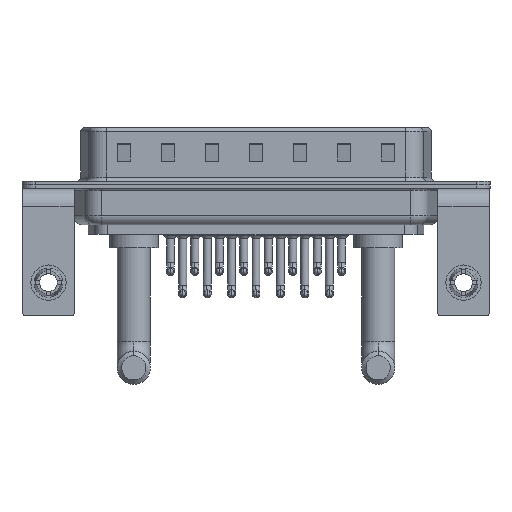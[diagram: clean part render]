
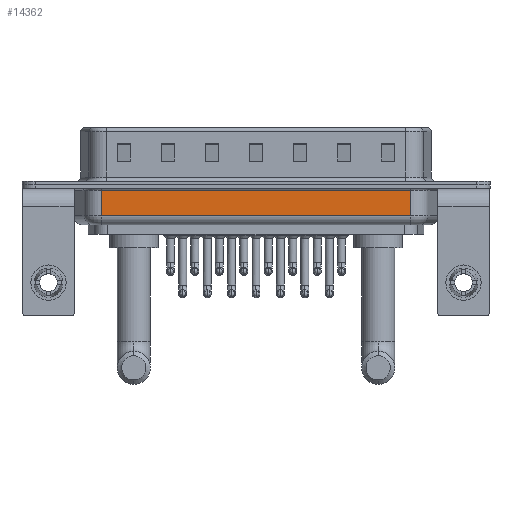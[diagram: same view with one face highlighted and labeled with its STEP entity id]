
A CAD part, front view. The second image highlights one B-rep face of the part: STEP entity #14362.
In plain terms, the highlighted planar face has unit normal (0, -1, 0).
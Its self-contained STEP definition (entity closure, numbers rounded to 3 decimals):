
#244 = CARTESIAN_POINT ( 'NONE',  ( 41.044, -5.35, -4.5 ) ) ;
#3924 = DIRECTION ( 'NONE',  ( 1., 0., 0. ) ) ;
#5867 = EDGE_CURVE ( 'NONE', #6937, #7468, #16823, .T. ) ;
#6099 = CARTESIAN_POINT ( 'NONE',  ( 6.006, -5.35, -3.5 ) ) ;
#6937 = VERTEX_POINT ( 'NONE', #19471 ) ;
#7468 = VERTEX_POINT ( 'NONE', #15445 ) ;
#7800 = LINE ( 'NONE', #26986, #19306 ) ;
#8134 = DIRECTION ( 'NONE',  ( -1., 0., 0. ) ) ;
#8943 = VECTOR ( 'NONE', #19300, 1000. ) ;
#9081 = EDGE_CURVE ( 'NONE', #18091, #7468, #10720, .T. ) ;
#10141 = AXIS2_PLACEMENT_3D ( 'NONE', #13619, #23970, #24506 ) ;
#10152 = CARTESIAN_POINT ( 'NONE',  ( 41.044, -5.35, -3.5 ) ) ;
#10720 = LINE ( 'NONE', #19139, #20099 ) ;
#12182 = ORIENTED_EDGE ( 'NONE', *, *, #18726, .T. ) ;
#13619 = CARTESIAN_POINT ( 'NONE',  ( 6.006, -5.35, -4.5 ) ) ;
#14362 = ADVANCED_FACE ( 'NONE', ( #24375 ), #24235, .F. ) ;
#14470 = VERTEX_POINT ( 'NONE', #10152 ) ;
#15445 = CARTESIAN_POINT ( 'NONE',  ( 6.006, -5.35, -0.65 ) ) ;
#15457 = ORIENTED_EDGE ( 'NONE', *, *, #9081, .F. ) ;
#16823 = LINE ( 'NONE', #19022, #17375 ) ;
#17375 = VECTOR ( 'NONE', #8134, 1000. ) ;
#18091 = VERTEX_POINT ( 'NONE', #6099 ) ;
#18463 = ORIENTED_EDGE ( 'NONE', *, *, #22312, .T. ) ;
#18726 = EDGE_CURVE ( 'NONE', #14470, #6937, #23853, .T. ) ;
#19022 = CARTESIAN_POINT ( 'NONE',  ( 6.006, -5.35, -0.65 ) ) ;
#19139 = CARTESIAN_POINT ( 'NONE',  ( 6.006, -5.35, -4.5 ) ) ;
#19300 = DIRECTION ( 'NONE',  ( 0., 0., 1. ) ) ;
#19306 = VECTOR ( 'NONE', #3924, 1000. ) ;
#19471 = CARTESIAN_POINT ( 'NONE',  ( 41.044, -5.35, -0.65 ) ) ;
#20099 = VECTOR ( 'NONE', #25482, 1000. ) ;
#22312 = EDGE_CURVE ( 'NONE', #18091, #14470, #7800, .T. ) ;
#23853 = LINE ( 'NONE', #244, #8943 ) ;
#23970 = DIRECTION ( 'NONE',  ( 0., 1., 0. ) ) ;
#24235 = PLANE ( 'NONE',  #10141 ) ;
#24375 = FACE_OUTER_BOUND ( 'NONE', #26123, .T. ) ;
#24506 = DIRECTION ( 'NONE',  ( 0., 0., 1. ) ) ;
#25482 = DIRECTION ( 'NONE',  ( 0., 0., 1. ) ) ;
#26123 = EDGE_LOOP ( 'NONE', ( #15457, #18463, #12182, #27138 ) ) ;
#26986 = CARTESIAN_POINT ( 'NONE',  ( 6.006, -5.35, -3.5 ) ) ;
#27138 = ORIENTED_EDGE ( 'NONE', *, *, #5867, .T. ) ;
